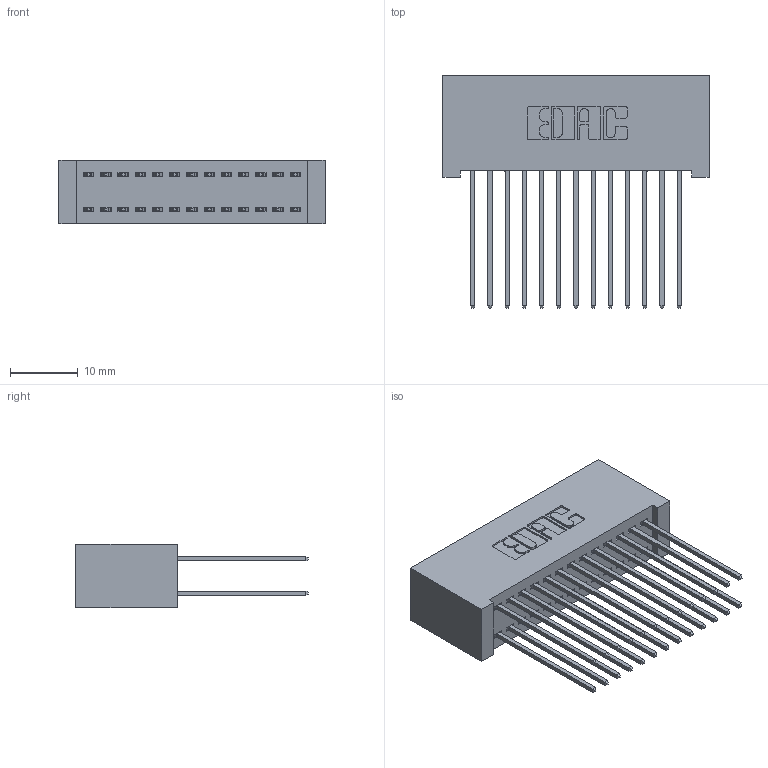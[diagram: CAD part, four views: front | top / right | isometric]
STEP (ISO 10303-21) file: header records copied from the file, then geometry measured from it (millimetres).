
FILE_DESCRIPTION (( 'STEP AP203' ), '1' );
FILE_NAME ('392-026-541-201.STEP', '2019-10-07T11:23:44', ( '' ), ( '' ), 'SwSTEP 2.0', 'SolidWorks 2016', '' );
FILE_SCHEMA (( 'CONFIG_CONTROL_DESIGN' ));
Length unit declared in the file: inch
Products named in the file (3): 342 Part_Lugless; 345-292-001_345-293-141; 392-026-541-201
Assembly tree (27 placements, depth 2):
  392-026-541-201
    342 Part_Lugless
    345-292-001_345-293-141  x26
Bounding box: 39.27 x 34.3 x 9.4 mm (x, y, z)
Volume: 3979.7 mm3; surface area: 6884.1 mm2
Topology: 27 solids, 27 shells, 1454 faces, 4305 edges, 2834 vertices
Faces by surface type: plane 998, cylinder 456
Entity records: 11723 total; most frequent: CARTESIAN_POINT 1974, ORIENTED_EDGE 1910, DIRECTION 1731, EDGE_CURVE 955, VECTOR 835, LINE 835, VERTEX_POINT 634, AXIS2_PLACEMENT_3D 448
